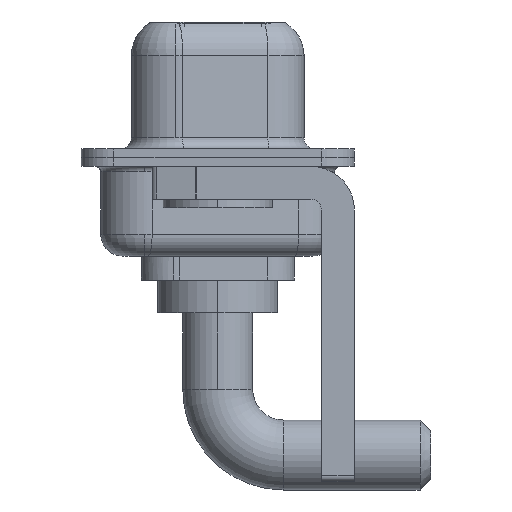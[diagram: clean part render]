
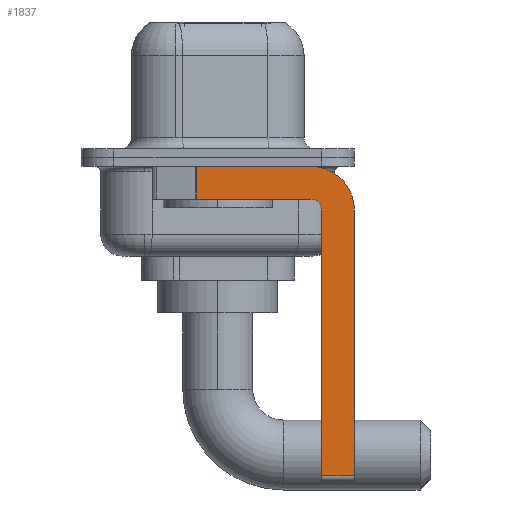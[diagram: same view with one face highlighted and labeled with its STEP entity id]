
A CAD part, left-side view. The second image highlights one B-rep face of the part: STEP entity #1837.
In plain terms, the highlighted planar face has unit normal (-1, 0, 0).
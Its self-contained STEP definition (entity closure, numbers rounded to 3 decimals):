
#101 = EDGE_CURVE ( 'NONE', #9907, #9647, #10169, .T. ) ;
#169 = EDGE_CURVE ( 'NONE', #530, #6886, #12312, .T. ) ;
#368 = ORIENTED_EDGE ( 'NONE', *, *, #739, .F. ) ;
#442 = CARTESIAN_POINT ( 'NONE',  ( -2.9, -4.75, -14.8 ) ) ;
#527 = CARTESIAN_POINT ( 'NONE',  ( -2.9, -4.25, -14.55 ) ) ;
#530 = VERTEX_POINT ( 'NONE', #8441 ) ;
#638 = VERTEX_POINT ( 'NONE', #3570 ) ;
#739 = EDGE_CURVE ( 'NONE', #638, #530, #10634, .T. ) ;
#1184 = CARTESIAN_POINT ( 'NONE',  ( -2.9, 0.978, -1.9 ) ) ;
#1195 = CARTESIAN_POINT ( 'NONE',  ( -2.9, -4.25, -2.4 ) ) ;
#1488 = CARTESIAN_POINT ( 'NONE',  ( -2.9, -6.25, -2.4 ) ) ;
#1638 = CARTESIAN_POINT ( 'NONE',  ( -2.9, -4.25, -1.9 ) ) ;
#1648 = DIRECTION ( 'NONE',  ( 1., 0., 0. ) ) ;
#1716 = CARTESIAN_POINT ( 'NONE',  ( -2.9, -4.25, -2.4 ) ) ;
#1781 = PLANE ( 'NONE',  #10307 ) ;
#1837 = ADVANCED_FACE ( 'NONE', ( #10042 ), #1781, .F. ) ;
#2213 = DIRECTION ( 'NONE',  ( 0., 0., 1. ) ) ;
#2287 = AXIS2_PLACEMENT_3D ( 'NONE', #1195, #10689, #2213 ) ;
#2648 = DIRECTION ( 'NONE',  ( 0., -1., 0. ) ) ;
#3014 = EDGE_CURVE ( 'NONE', #9647, #8678, #4620, .T. ) ;
#3040 = VECTOR ( 'NONE', #6767, 1000. ) ;
#3145 = CARTESIAN_POINT ( 'NONE',  ( -2.9, -6.25, -2.4 ) ) ;
#3175 = ORIENTED_EDGE ( 'NONE', *, *, #3014, .F. ) ;
#3318 = ORIENTED_EDGE ( 'NONE', *, *, #169, .F. ) ;
#3538 = LINE ( 'NONE', #4507, #3040 ) ;
#3570 = CARTESIAN_POINT ( 'NONE',  ( -2.9, -4.75, -14.55 ) ) ;
#3663 = CARTESIAN_POINT ( 'NONE',  ( -2.9, -4.25, -0.4 ) ) ;
#4034 = DIRECTION ( 'NONE',  ( 0., 0., -1. ) ) ;
#4386 = EDGE_CURVE ( 'NONE', #9907, #6169, #3538, .T. ) ;
#4507 = CARTESIAN_POINT ( 'NONE',  ( -2.9, 0.978, -1.9 ) ) ;
#4620 = CIRCLE ( 'NONE', #8110, 2. ) ;
#4779 = DIRECTION ( 'NONE',  ( 0., 0., -1. ) ) ;
#5071 = VECTOR ( 'NONE', #2648, 1000. ) ;
#5357 = EDGE_LOOP ( 'NONE', ( #12181, #12950, #8508, #3318, #368, #12516, #6650, #3175 ) ) ;
#5579 = EDGE_CURVE ( 'NONE', #638, #7816, #6609, .T. ) ;
#6169 = VERTEX_POINT ( 'NONE', #1184 ) ;
#6538 = CARTESIAN_POINT ( 'NONE',  ( -2.9, 0.978, -0.4 ) ) ;
#6609 = LINE ( 'NONE', #527, #10067 ) ;
#6650 = ORIENTED_EDGE ( 'NONE', *, *, #12396, .F. ) ;
#6767 = DIRECTION ( 'NONE',  ( 0., 0., -1. ) ) ;
#6886 = VERTEX_POINT ( 'NONE', #9830 ) ;
#6898 = DIRECTION ( 'NONE',  ( 0., 0., -1. ) ) ;
#7164 = CARTESIAN_POINT ( 'NONE',  ( -2.9, -6.25, -14.55 ) ) ;
#7321 = LINE ( 'NONE', #3145, #10405 ) ;
#7764 = LINE ( 'NONE', #1638, #10125 ) ;
#7816 = VERTEX_POINT ( 'NONE', #7164 ) ;
#8110 = AXIS2_PLACEMENT_3D ( 'NONE', #1716, #11944, #6898 ) ;
#8243 = EDGE_CURVE ( 'NONE', #6886, #6169, #7764, .T. ) ;
#8441 = CARTESIAN_POINT ( 'NONE',  ( -2.9, -4.75, -2.4 ) ) ;
#8508 = ORIENTED_EDGE ( 'NONE', *, *, #8243, .F. ) ;
#8678 = VERTEX_POINT ( 'NONE', #1488 ) ;
#8722 = DIRECTION ( 'NONE',  ( 0., -1., 0. ) ) ;
#9647 = VERTEX_POINT ( 'NONE', #3663 ) ;
#9830 = CARTESIAN_POINT ( 'NONE',  ( -2.9, -4.25, -1.9 ) ) ;
#9907 = VERTEX_POINT ( 'NONE', #6538 ) ;
#10032 = DIRECTION ( 'NONE',  ( 0., 1., 0. ) ) ;
#10042 = FACE_OUTER_BOUND ( 'NONE', #5357, .T. ) ;
#10067 = VECTOR ( 'NONE', #8722, 1000. ) ;
#10125 = VECTOR ( 'NONE', #10032, 1000. ) ;
#10169 = LINE ( 'NONE', #11050, #5071 ) ;
#10307 = AXIS2_PLACEMENT_3D ( 'NONE', #10997, #1648, #4779 ) ;
#10405 = VECTOR ( 'NONE', #4034, 1000. ) ;
#10634 = LINE ( 'NONE', #442, #10920 ) ;
#10689 = DIRECTION ( 'NONE',  ( -1., 0., 0. ) ) ;
#10920 = VECTOR ( 'NONE', #11701, 1000. ) ;
#10997 = CARTESIAN_POINT ( 'NONE',  ( -2.9, -4.25, -2.4 ) ) ;
#11050 = CARTESIAN_POINT ( 'NONE',  ( -2.9, 3., -0.4 ) ) ;
#11701 = DIRECTION ( 'NONE',  ( 0., 0., 1. ) ) ;
#11944 = DIRECTION ( 'NONE',  ( 1., 0., 0. ) ) ;
#12181 = ORIENTED_EDGE ( 'NONE', *, *, #101, .F. ) ;
#12312 = CIRCLE ( 'NONE', #2287, 0.5 ) ;
#12396 = EDGE_CURVE ( 'NONE', #8678, #7816, #7321, .T. ) ;
#12516 = ORIENTED_EDGE ( 'NONE', *, *, #5579, .T. ) ;
#12950 = ORIENTED_EDGE ( 'NONE', *, *, #4386, .T. ) ;
